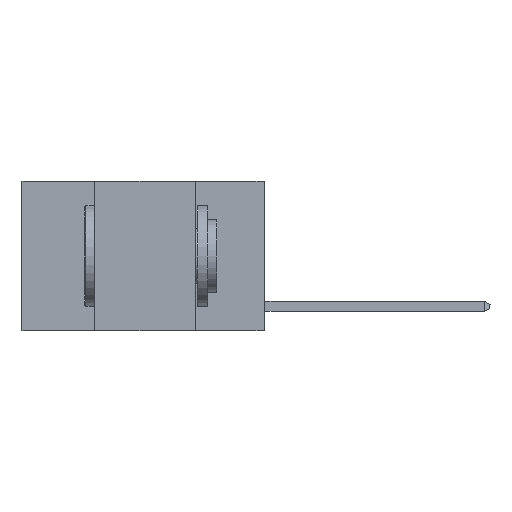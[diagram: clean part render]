
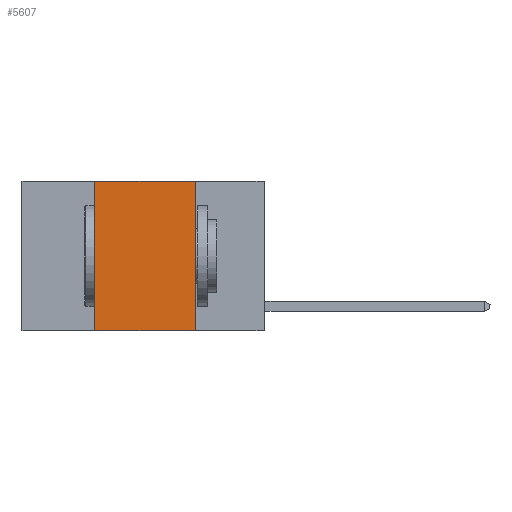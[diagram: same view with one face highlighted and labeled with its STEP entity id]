
A CAD part, left-side view. The second image highlights one B-rep face of the part: STEP entity #5607.
In plain terms, the highlighted planar face has unit normal (-1, 0, 0).
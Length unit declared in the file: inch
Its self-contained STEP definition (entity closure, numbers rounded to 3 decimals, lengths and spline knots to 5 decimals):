
#218 = DIRECTION ( 'NONE',  ( 0., 0., -1. ) ) ;
#248 = DIRECTION ( 'NONE',  ( 0., 0., -1. ) ) ;
#862 = EDGE_CURVE ( 'NONE', #2424, #4499, #6656, .T. ) ;
#864 = VERTEX_POINT ( 'NONE', #9643 ) ;
#1662 = DIRECTION ( 'NONE',  ( 1., 0., 0. ) ) ;
#1823 = CARTESIAN_POINT ( 'NONE',  ( 0., 0.17, 0. ) ) ;
#1896 = VERTEX_POINT ( 'NONE', #3005 ) ;
#2144 = CARTESIAN_POINT ( 'NONE',  ( 0., 0.6, 0. ) ) ;
#2360 = VECTOR ( 'NONE', #4300, 39.37008 ) ;
#2389 = AXIS2_PLACEMENT_3D ( 'NONE', #7663, #1662, #218 ) ;
#2424 = VERTEX_POINT ( 'NONE', #2837 ) ;
#2837 = CARTESIAN_POINT ( 'NONE',  ( 0., 0.42, -0.37 ) ) ;
#3005 = CARTESIAN_POINT ( 'NONE',  ( 0., 0.17, 0. ) ) ;
#3440 = CARTESIAN_POINT ( 'NONE',  ( 0., 0.42, 0. ) ) ;
#3615 = CARTESIAN_POINT ( 'NONE',  ( 0., 0.42, 0. ) ) ;
#4126 = EDGE_LOOP ( 'NONE', ( #9554, #5268, #6142, #6942 ) ) ;
#4300 = DIRECTION ( 'NONE',  ( 0., 0., 1. ) ) ;
#4456 = DIRECTION ( 'NONE',  ( 0., -1., 0. ) ) ;
#4499 = VERTEX_POINT ( 'NONE', #3615 ) ;
#4549 = FACE_OUTER_BOUND ( 'NONE', #4126, .T. ) ;
#4906 = LINE ( 'NONE', #2144, #5391 ) ;
#5268 = ORIENTED_EDGE ( 'NONE', *, *, #6550, .F. ) ;
#5344 = LINE ( 'NONE', #7240, #9753 ) ;
#5391 = VECTOR ( 'NONE', #4456, 39.37008 ) ;
#5607 = ADVANCED_FACE ( 'NONE', ( #4549 ), #7776, .F. ) ;
#6142 = ORIENTED_EDGE ( 'NONE', *, *, #862, .F. ) ;
#6156 = VECTOR ( 'NONE', #248, 39.37008 ) ;
#6550 = EDGE_CURVE ( 'NONE', #4499, #1896, #4906, .T. ) ;
#6656 = LINE ( 'NONE', #3440, #2360 ) ;
#6796 = EDGE_CURVE ( 'NONE', #1896, #864, #8130, .T. ) ;
#6942 = ORIENTED_EDGE ( 'NONE', *, *, #7957, .T. ) ;
#7240 = CARTESIAN_POINT ( 'NONE',  ( 0., 0.6, -0.37 ) ) ;
#7663 = CARTESIAN_POINT ( 'NONE',  ( 0., 0.6, 0. ) ) ;
#7776 = PLANE ( 'NONE',  #2389 ) ;
#7957 = EDGE_CURVE ( 'NONE', #2424, #864, #5344, .T. ) ;
#8130 = LINE ( 'NONE', #1823, #6156 ) ;
#9554 = ORIENTED_EDGE ( 'NONE', *, *, #6796, .F. ) ;
#9566 = DIRECTION ( 'NONE',  ( 0., -1., 0. ) ) ;
#9643 = CARTESIAN_POINT ( 'NONE',  ( 0., 0.17, -0.37 ) ) ;
#9753 = VECTOR ( 'NONE', #9566, 39.37008 ) ;
